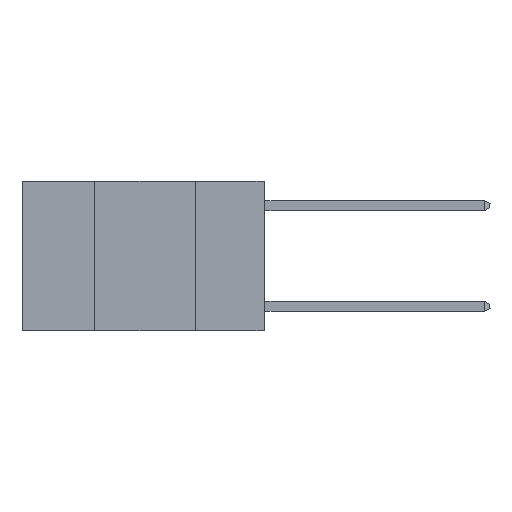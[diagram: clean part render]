
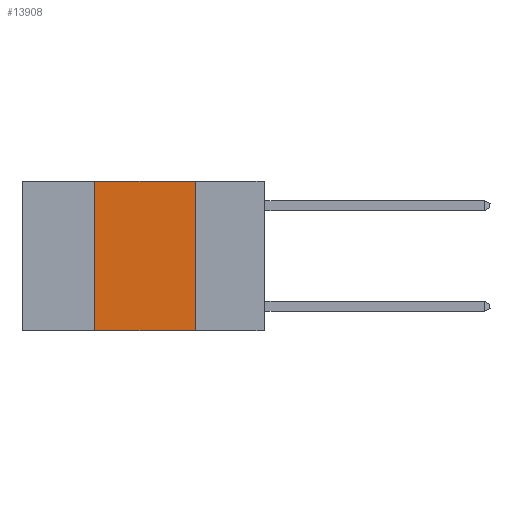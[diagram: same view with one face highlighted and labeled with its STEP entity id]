
A CAD part, left-side view. The second image highlights one B-rep face of the part: STEP entity #13908.
In plain terms, the highlighted planar face has unit normal (-1, 0, 0).
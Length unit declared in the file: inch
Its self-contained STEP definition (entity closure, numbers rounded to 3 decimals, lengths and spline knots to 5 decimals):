
#191 = ORIENTED_EDGE ( 'NONE', *, *, #7038, .F. ) ;
#916 = CARTESIAN_POINT ( 'NONE',  ( 0., 0.42, 0. ) ) ;
#989 = AXIS2_PLACEMENT_3D ( 'NONE', #9589, #3820, #8452 ) ;
#1168 = VERTEX_POINT ( 'NONE', #11501 ) ;
#1929 = VECTOR ( 'NONE', #7873, 39.37008 ) ;
#2412 = VERTEX_POINT ( 'NONE', #5308 ) ;
#2874 = ORIENTED_EDGE ( 'NONE', *, *, #15014, .T. ) ;
#3301 = VECTOR ( 'NONE', #8916, 39.37008 ) ;
#3706 = VECTOR ( 'NONE', #12541, 39.37008 ) ;
#3820 = DIRECTION ( 'NONE',  ( 1., 0., 0. ) ) ;
#4290 = CARTESIAN_POINT ( 'NONE',  ( 0., 0.6, 0. ) ) ;
#4360 = EDGE_LOOP ( 'NONE', ( #9632, #191, #7738, #2874 ) ) ;
#4962 = PLANE ( 'NONE',  #989 ) ;
#5214 = EDGE_CURVE ( 'NONE', #1168, #14575, #5434, .T. ) ;
#5308 = CARTESIAN_POINT ( 'NONE',  ( 0., 0.17, 0. ) ) ;
#5434 = LINE ( 'NONE', #916, #3706 ) ;
#5570 = LINE ( 'NONE', #4290, #3301 ) ;
#6995 = LINE ( 'NONE', #10336, #9784 ) ;
#7038 = EDGE_CURVE ( 'NONE', #14575, #2412, #5570, .T. ) ;
#7738 = ORIENTED_EDGE ( 'NONE', *, *, #5214, .F. ) ;
#7873 = DIRECTION ( 'NONE',  ( 0., 0., -1. ) ) ;
#8009 = DIRECTION ( 'NONE',  ( 0., -1., 0. ) ) ;
#8225 = VERTEX_POINT ( 'NONE', #10953 ) ;
#8452 = DIRECTION ( 'NONE',  ( 0., 0., -1. ) ) ;
#8872 = CARTESIAN_POINT ( 'NONE',  ( 0., 0.17, 0. ) ) ;
#8916 = DIRECTION ( 'NONE',  ( 0., -1., 0. ) ) ;
#9534 = CARTESIAN_POINT ( 'NONE',  ( 0., 0.42, 0. ) ) ;
#9589 = CARTESIAN_POINT ( 'NONE',  ( 0., 0.6, 0. ) ) ;
#9632 = ORIENTED_EDGE ( 'NONE', *, *, #11653, .F. ) ;
#9784 = VECTOR ( 'NONE', #8009, 39.37008 ) ;
#10336 = CARTESIAN_POINT ( 'NONE',  ( 0., 0.6, -0.37 ) ) ;
#10691 = FACE_OUTER_BOUND ( 'NONE', #4360, .T. ) ;
#10953 = CARTESIAN_POINT ( 'NONE',  ( 0., 0.17, -0.37 ) ) ;
#11335 = LINE ( 'NONE', #8872, #1929 ) ;
#11501 = CARTESIAN_POINT ( 'NONE',  ( 0., 0.42, -0.37 ) ) ;
#11653 = EDGE_CURVE ( 'NONE', #2412, #8225, #11335, .T. ) ;
#12541 = DIRECTION ( 'NONE',  ( 0., 0., 1. ) ) ;
#13908 = ADVANCED_FACE ( 'NONE', ( #10691 ), #4962, .F. ) ;
#14575 = VERTEX_POINT ( 'NONE', #9534 ) ;
#15014 = EDGE_CURVE ( 'NONE', #1168, #8225, #6995, .T. ) ;
